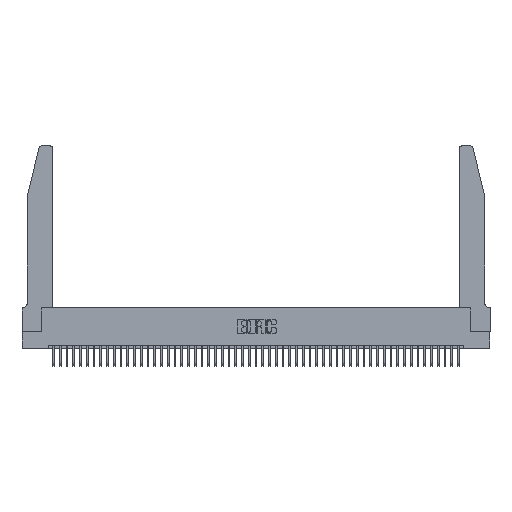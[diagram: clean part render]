
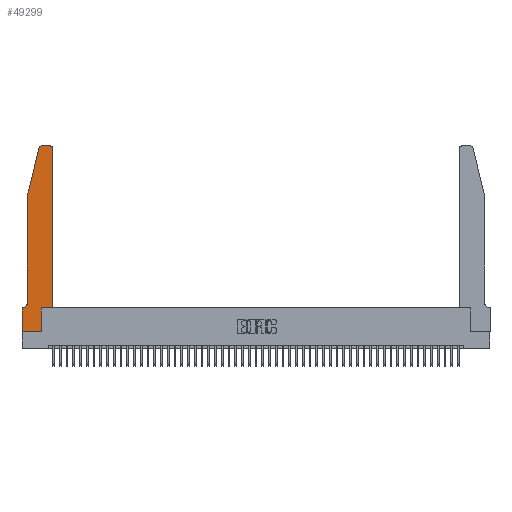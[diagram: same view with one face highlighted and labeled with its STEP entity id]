
A CAD part, top view. The second image highlights one B-rep face of the part: STEP entity #49299.
In plain terms, the highlighted planar face has unit normal (0, 0, 1).
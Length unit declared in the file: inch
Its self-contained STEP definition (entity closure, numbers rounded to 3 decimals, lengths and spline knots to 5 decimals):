
#51 = CARTESIAN_POINT ( 'NONE',  ( 0.0755, 2., 0.37 ) ) ;
#341 = VERTEX_POINT ( 'NONE', #44599 ) ;
#361 = VERTEX_POINT ( 'NONE', #41156 ) ;
#371 = ORIENTED_EDGE ( 'NONE', *, *, #10621, .T. ) ;
#473 = ORIENTED_EDGE ( 'NONE', *, *, #44813, .T. ) ;
#1539 = VERTEX_POINT ( 'NONE', #4894 ) ;
#2116 = DIRECTION ( 'NONE',  ( 1., 0., 0. ) ) ;
#3070 = DIRECTION ( 'NONE',  ( 0., 1., 0. ) ) ;
#3158 = LINE ( 'NONE', #31841, #45647 ) ;
#3248 = VECTOR ( 'NONE', #40706, 39.37008 ) ;
#3481 = EDGE_CURVE ( 'NONE', #25155, #341, #4547, .T. ) ;
#3873 = DIRECTION ( 'NONE',  ( 0., -1., 0. ) ) ;
#4352 = ORIENTED_EDGE ( 'NONE', *, *, #3481, .T. ) ;
#4547 = LINE ( 'NONE', #12859, #3248 ) ;
#4737 = CARTESIAN_POINT ( 'NONE',  ( 0.0055, 0.42, 0.37 ) ) ;
#4784 = CARTESIAN_POINT ( 'NONE',  ( 0., 0., 0.37 ) ) ;
#4894 = CARTESIAN_POINT ( 'NONE',  ( 0.25487, 2.72718, 0.37 ) ) ;
#5632 = FACE_OUTER_BOUND ( 'NONE', #28175, .T. ) ;
#5659 = VERTEX_POINT ( 'NONE', #28972 ) ;
#5860 = EDGE_CURVE ( 'NONE', #31142, #50555, #16238, .T. ) ;
#6288 = ORIENTED_EDGE ( 'NONE', *, *, #36294, .T. ) ;
#7043 = CARTESIAN_POINT ( 'NONE',  ( 0.4505, 2.72, 0.37 ) ) ;
#8207 = VECTOR ( 'NONE', #3070, 39.37008 ) ;
#8609 = EDGE_CURVE ( 'NONE', #5659, #33874, #39621, .T. ) ;
#8854 = DIRECTION ( 'NONE',  ( -1., 0., 0. ) ) ;
#10621 = EDGE_CURVE ( 'NONE', #1539, #40378, #10764, .T. ) ;
#10698 = VECTOR ( 'NONE', #32720, 39.37008 ) ;
#10764 = LINE ( 'NONE', #12452, #51736 ) ;
#10797 = ORIENTED_EDGE ( 'NONE', *, *, #48602, .T. ) ;
#10985 = CARTESIAN_POINT ( 'NONE',  ( 0.0055, 0.35, 0.37 ) ) ;
#11231 = EDGE_CURVE ( 'NONE', #16564, #31142, #26341, .T. ) ;
#12246 = CARTESIAN_POINT ( 'NONE',  ( 0.4505, 0.35, 0.37 ) ) ;
#12452 = CARTESIAN_POINT ( 'NONE',  ( 0.0755, 2., 0.37 ) ) ;
#12582 = CIRCLE ( 'NONE', #44169, 0.03 ) ;
#12859 = CARTESIAN_POINT ( 'NONE',  ( 0.0755, 0.35, 0.37 ) ) ;
#15609 = DIRECTION ( 'NONE',  ( 0., 0., 1. ) ) ;
#15744 = VECTOR ( 'NONE', #35885, 39.37008 ) ;
#16238 = LINE ( 'NONE', #18175, #36151 ) ;
#16564 = VERTEX_POINT ( 'NONE', #29442 ) ;
#17216 = AXIS2_PLACEMENT_3D ( 'NONE', #43897, #20088, #47893 ) ;
#17650 = ORIENTED_EDGE ( 'NONE', *, *, #5860, .T. ) ;
#18109 = VERTEX_POINT ( 'NONE', #22990 ) ;
#18175 = CARTESIAN_POINT ( 'NONE',  ( 0.4505, 0.35, 0.37 ) ) ;
#18771 = VERTEX_POINT ( 'NONE', #7043 ) ;
#18981 = EDGE_CURVE ( 'NONE', #40378, #18109, #49686, .T. ) ;
#19406 = AXIS2_PLACEMENT_3D ( 'NONE', #4737, #32668, #8854 ) ;
#19726 = CARTESIAN_POINT ( 'NONE',  ( 0.284, 2.72, 0.37 ) ) ;
#20088 = DIRECTION ( 'NONE',  ( 0., 0., 1. ) ) ;
#20711 = ORIENTED_EDGE ( 'NONE', *, *, #11231, .T. ) ;
#22497 = EDGE_CURVE ( 'NONE', #18771, #5659, #35183, .T. ) ;
#22990 = CARTESIAN_POINT ( 'NONE',  ( 0.0755, 0.42, 0.37 ) ) ;
#23708 = DIRECTION ( 'NONE',  ( 1., 0., 0. ) ) ;
#25155 = VERTEX_POINT ( 'NONE', #10985 ) ;
#25550 = ORIENTED_EDGE ( 'NONE', *, *, #18981, .T. ) ;
#26341 = LINE ( 'NONE', #31860, #15744 ) ;
#27283 = AXIS2_PLACEMENT_3D ( 'NONE', #39469, #15609, #43445 ) ;
#27933 = DIRECTION ( 'NONE',  ( -1., 0., 0. ) ) ;
#28175 = EDGE_LOOP ( 'NONE', ( #48537, #41768, #371, #25550, #473, #4352, #47436, #6288, #20711, #17650, #10797, #31923 ) ) ;
#28239 = CARTESIAN_POINT ( 'NONE',  ( 0.2865, 0.35, 0.37 ) ) ;
#28573 = VECTOR ( 'NONE', #44977, 39.37008 ) ;
#28972 = CARTESIAN_POINT ( 'NONE',  ( 0.4205, 2.75, 0.37 ) ) ;
#29021 = VECTOR ( 'NONE', #27933, 39.37008 ) ;
#29442 = CARTESIAN_POINT ( 'NONE',  ( 0.2865, 0., 0.37 ) ) ;
#31142 = VERTEX_POINT ( 'NONE', #28239 ) ;
#31813 = LINE ( 'NONE', #4784, #10698 ) ;
#31841 = CARTESIAN_POINT ( 'NONE',  ( 0., 0., 0.37 ) ) ;
#31860 = CARTESIAN_POINT ( 'NONE',  ( 0.2865, 0.35, 0.37 ) ) ;
#31894 = PLANE ( 'NONE',  #17216 ) ;
#31923 = ORIENTED_EDGE ( 'NONE', *, *, #22497, .T. ) ;
#32668 = DIRECTION ( 'NONE',  ( 0., 0., -1. ) ) ;
#32720 = DIRECTION ( 'NONE',  ( 1., 0., 0. ) ) ;
#33874 = VERTEX_POINT ( 'NONE', #46461 ) ;
#35183 = CIRCLE ( 'NONE', #27283, 0.03 ) ;
#35885 = DIRECTION ( 'NONE',  ( 0., 1., 0. ) ) ;
#36068 = EDGE_CURVE ( 'NONE', #33874, #1539, #12582, .T. ) ;
#36151 = VECTOR ( 'NONE', #2116, 39.37008 ) ;
#36279 = DIRECTION ( 'NONE',  ( -0.239, -0.971, 0. ) ) ;
#36294 = EDGE_CURVE ( 'NONE', #361, #16564, #31813, .T. ) ;
#37538 = LINE ( 'NONE', #43085, #8207 ) ;
#39469 = CARTESIAN_POINT ( 'NONE',  ( 0.4205, 2.72, 0.37 ) ) ;
#39621 = LINE ( 'NONE', #51655, #29021 ) ;
#40378 = VERTEX_POINT ( 'NONE', #51 ) ;
#40706 = DIRECTION ( 'NONE',  ( -1., 0., 0. ) ) ;
#41027 = CARTESIAN_POINT ( 'NONE',  ( 0.0755, 2., 0.37 ) ) ;
#41156 = CARTESIAN_POINT ( 'NONE',  ( 0., 0., 0.37 ) ) ;
#41768 = ORIENTED_EDGE ( 'NONE', *, *, #36068, .T. ) ;
#42621 = EDGE_CURVE ( 'NONE', #341, #361, #3158, .T. ) ;
#43085 = CARTESIAN_POINT ( 'NONE',  ( 0.4505, 0.35, 0.37 ) ) ;
#43445 = DIRECTION ( 'NONE',  ( 1., 0., 0. ) ) ;
#43897 = CARTESIAN_POINT ( 'NONE',  ( 0., 0.35, 0.37 ) ) ;
#44169 = AXIS2_PLACEMENT_3D ( 'NONE', #19726, #47519, #23708 ) ;
#44599 = CARTESIAN_POINT ( 'NONE',  ( 0., 0.35, 0.37 ) ) ;
#44813 = EDGE_CURVE ( 'NONE', #18109, #25155, #50933, .T. ) ;
#44977 = DIRECTION ( 'NONE',  ( 0., -1., 0. ) ) ;
#45647 = VECTOR ( 'NONE', #3873, 39.37008 ) ;
#46461 = CARTESIAN_POINT ( 'NONE',  ( 0.284, 2.75, 0.37 ) ) ;
#47436 = ORIENTED_EDGE ( 'NONE', *, *, #42621, .T. ) ;
#47519 = DIRECTION ( 'NONE',  ( 0., 0., 1. ) ) ;
#47893 = DIRECTION ( 'NONE',  ( 1., 0., 0. ) ) ;
#48537 = ORIENTED_EDGE ( 'NONE', *, *, #8609, .T. ) ;
#48602 = EDGE_CURVE ( 'NONE', #50555, #18771, #37538, .T. ) ;
#49299 = ADVANCED_FACE ( 'NONE', ( #5632 ), #31894, .T. ) ;
#49686 = LINE ( 'NONE', #41027, #28573 ) ;
#50555 = VERTEX_POINT ( 'NONE', #12246 ) ;
#50933 = CIRCLE ( 'NONE', #19406, 0.07 ) ;
#51655 = CARTESIAN_POINT ( 'NONE',  ( 0.2605, 2.75, 0.37 ) ) ;
#51736 = VECTOR ( 'NONE', #36279, 39.37008 ) ;
